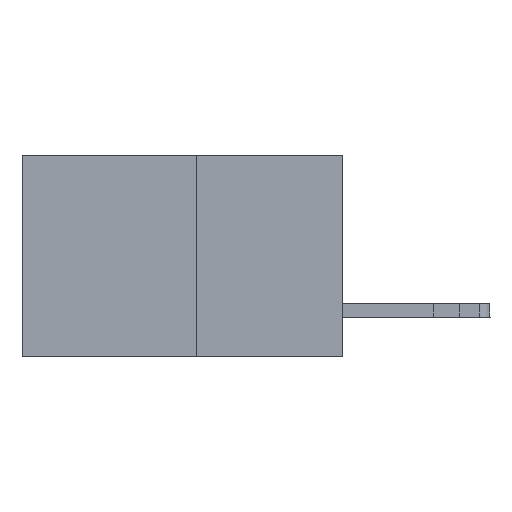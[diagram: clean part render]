
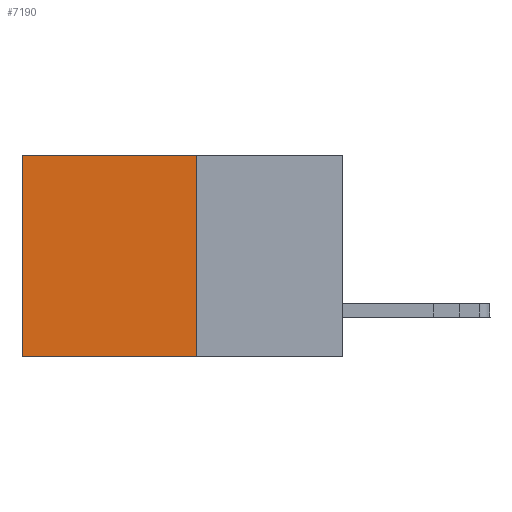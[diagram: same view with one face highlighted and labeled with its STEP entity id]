
A CAD part, left-side view. The second image highlights one B-rep face of the part: STEP entity #7190.
In plain terms, the highlighted planar face has unit normal (-1, 0, 0).
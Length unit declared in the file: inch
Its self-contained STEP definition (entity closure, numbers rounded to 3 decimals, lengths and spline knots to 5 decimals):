
#430 = VERTEX_POINT ( 'NONE', #11223 ) ;
#605 = FACE_OUTER_BOUND ( 'NONE', #2787, .T. ) ;
#817 = VERTEX_POINT ( 'NONE', #2865 ) ;
#2688 = LINE ( 'NONE', #11558, #13150 ) ;
#2787 = EDGE_LOOP ( 'NONE', ( #13520, #17613, #16066, #4339 ) ) ;
#2865 = CARTESIAN_POINT ( 'NONE',  ( 0.277, 0.27, 0. ) ) ;
#4339 = ORIENTED_EDGE ( 'NONE', *, *, #17144, .T. ) ;
#4472 = DIRECTION ( 'NONE',  ( 0., 0., -1. ) ) ;
#4824 = DIRECTION ( 'NONE',  ( 0., 0., -1. ) ) ;
#5012 = LINE ( 'NONE', #10708, #5250 ) ;
#5250 = VECTOR ( 'NONE', #16395, 39.37008 ) ;
#5796 = EDGE_CURVE ( 'NONE', #16634, #430, #10052, .T. ) ;
#7190 = ADVANCED_FACE ( 'NONE', ( #605 ), #12516, .F. ) ;
#7231 = EDGE_CURVE ( 'NONE', #17716, #430, #5012, .T. ) ;
#8152 = CARTESIAN_POINT ( 'NONE',  ( 0.277, 0.27, -0.37 ) ) ;
#8593 = DIRECTION ( 'NONE',  ( 0., 1., 0. ) ) ;
#10052 = LINE ( 'NONE', #15824, #13656 ) ;
#10708 = CARTESIAN_POINT ( 'NONE',  ( 0.277, 0.27, -0.37 ) ) ;
#10915 = AXIS2_PLACEMENT_3D ( 'NONE', #8152, #12093, #4824 ) ;
#11223 = CARTESIAN_POINT ( 'NONE',  ( 0.277, 0.59, -0.37 ) ) ;
#11289 = CARTESIAN_POINT ( 'NONE',  ( 0.277, 0.27, -0.37 ) ) ;
#11558 = CARTESIAN_POINT ( 'NONE',  ( 0.277, 0.27, 0. ) ) ;
#12093 = DIRECTION ( 'NONE',  ( 1., 0., 0. ) ) ;
#12516 = PLANE ( 'NONE',  #10915 ) ;
#13150 = VECTOR ( 'NONE', #8593, 39.37008 ) ;
#13520 = ORIENTED_EDGE ( 'NONE', *, *, #5796, .T. ) ;
#13656 = VECTOR ( 'NONE', #15728, 39.37008 ) ;
#14267 = LINE ( 'NONE', #11289, #17955 ) ;
#14513 = CARTESIAN_POINT ( 'NONE',  ( 0.277, 0.27, -0.37 ) ) ;
#15728 = DIRECTION ( 'NONE',  ( 0., 0., -1. ) ) ;
#15824 = CARTESIAN_POINT ( 'NONE',  ( 0.277, 0.59, -0.37 ) ) ;
#16066 = ORIENTED_EDGE ( 'NONE', *, *, #17171, .F. ) ;
#16333 = CARTESIAN_POINT ( 'NONE',  ( 0.277, 0.59, 0. ) ) ;
#16395 = DIRECTION ( 'NONE',  ( 0., 1., 0. ) ) ;
#16634 = VERTEX_POINT ( 'NONE', #16333 ) ;
#17144 = EDGE_CURVE ( 'NONE', #817, #16634, #2688, .T. ) ;
#17171 = EDGE_CURVE ( 'NONE', #817, #17716, #14267, .T. ) ;
#17613 = ORIENTED_EDGE ( 'NONE', *, *, #7231, .F. ) ;
#17716 = VERTEX_POINT ( 'NONE', #14513 ) ;
#17955 = VECTOR ( 'NONE', #4472, 39.37008 ) ;
